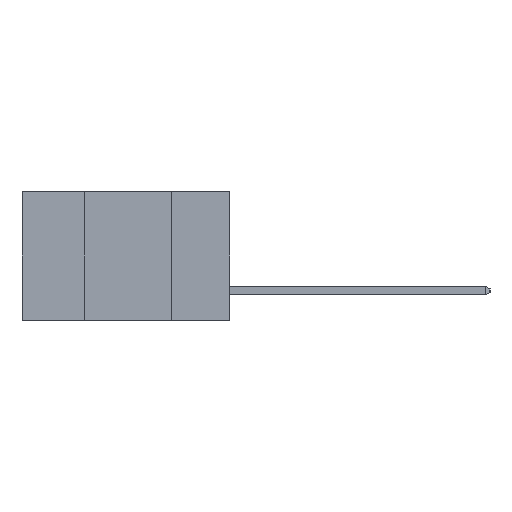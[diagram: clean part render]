
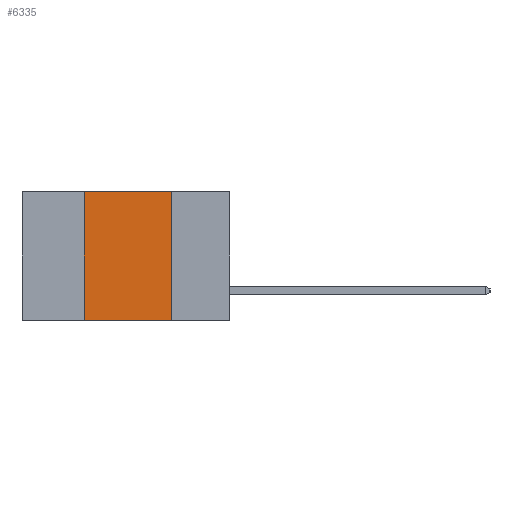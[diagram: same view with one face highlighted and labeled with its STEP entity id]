
A CAD part, left-side view. The second image highlights one B-rep face of the part: STEP entity #6335.
In plain terms, the highlighted planar face has unit normal (-1, 0, 0).
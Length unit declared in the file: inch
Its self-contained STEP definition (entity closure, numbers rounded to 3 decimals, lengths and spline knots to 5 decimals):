
#1959 = EDGE_CURVE ( 'NONE', #7969, #22691, #22891, .T. ) ;
#2859 = LINE ( 'NONE', #3634, #22865 ) ;
#3467 = DIRECTION ( 'NONE',  ( 0., 0., 1. ) ) ;
#3634 = CARTESIAN_POINT ( 'NONE',  ( 0., 0.42, -0.37 ) ) ;
#5433 = ORIENTED_EDGE ( 'NONE', *, *, #6060, .T. ) ;
#6060 = EDGE_CURVE ( 'NONE', #23528, #10393, #12592, .T. ) ;
#6085 = VECTOR ( 'NONE', #22548, 39.37008 ) ;
#6335 = ADVANCED_FACE ( 'NONE', ( #20982 ), #7133, .F. ) ;
#6650 = ORIENTED_EDGE ( 'NONE', *, *, #15750, .F. ) ;
#6692 = LINE ( 'NONE', #23577, #6085 ) ;
#7083 = DIRECTION ( 'NONE',  ( 0., 0., -1. ) ) ;
#7103 = DIRECTION ( 'NONE',  ( 1., 0., 0. ) ) ;
#7133 = PLANE ( 'NONE',  #17147 ) ;
#7357 = CARTESIAN_POINT ( 'NONE',  ( 0., 0.6, 0. ) ) ;
#7969 = VERTEX_POINT ( 'NONE', #16836 ) ;
#8766 = ORIENTED_EDGE ( 'NONE', *, *, #1959, .F. ) ;
#10393 = VERTEX_POINT ( 'NONE', #14138 ) ;
#10625 = CARTESIAN_POINT ( 'NONE',  ( 0., 0.6, -0.37 ) ) ;
#10633 = DIRECTION ( 'NONE',  ( 0., -1., 0. ) ) ;
#10699 = EDGE_CURVE ( 'NONE', #22691, #10393, #6692, .T. ) ;
#12592 = LINE ( 'NONE', #10625, #17525 ) ;
#13151 = VECTOR ( 'NONE', #23415, 39.37008 ) ;
#14138 = CARTESIAN_POINT ( 'NONE',  ( 0., 0.17, -0.37 ) ) ;
#14387 = CARTESIAN_POINT ( 'NONE',  ( 0., 0.6, 0. ) ) ;
#14435 = EDGE_LOOP ( 'NONE', ( #19874, #8766, #6650, #5433 ) ) ;
#15750 = EDGE_CURVE ( 'NONE', #23528, #7969, #2859, .T. ) ;
#16836 = CARTESIAN_POINT ( 'NONE',  ( 0., 0.42, 0. ) ) ;
#17147 = AXIS2_PLACEMENT_3D ( 'NONE', #7357, #7103, #7083 ) ;
#17475 = CARTESIAN_POINT ( 'NONE',  ( 0., 0.42, -0.37 ) ) ;
#17525 = VECTOR ( 'NONE', #10633, 39.37008 ) ;
#18411 = CARTESIAN_POINT ( 'NONE',  ( 0., 0.17, 0. ) ) ;
#19874 = ORIENTED_EDGE ( 'NONE', *, *, #10699, .F. ) ;
#20982 = FACE_OUTER_BOUND ( 'NONE', #14435, .T. ) ;
#22548 = DIRECTION ( 'NONE',  ( 0., 0., -1. ) ) ;
#22691 = VERTEX_POINT ( 'NONE', #18411 ) ;
#22865 = VECTOR ( 'NONE', #3467, 39.37008 ) ;
#22891 = LINE ( 'NONE', #14387, #13151 ) ;
#23415 = DIRECTION ( 'NONE',  ( 0., -1., 0. ) ) ;
#23528 = VERTEX_POINT ( 'NONE', #17475 ) ;
#23577 = CARTESIAN_POINT ( 'NONE',  ( 0., 0.17, -0.37 ) ) ;
